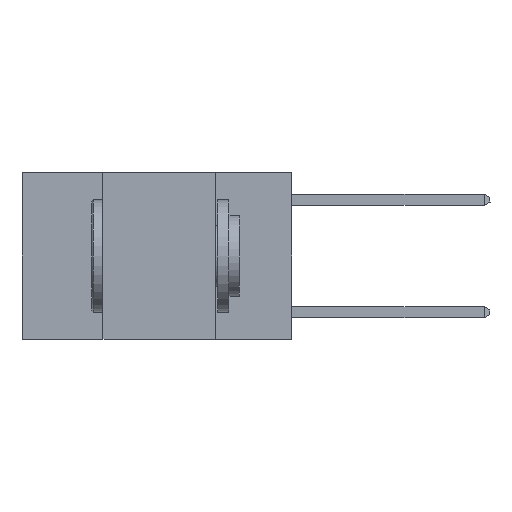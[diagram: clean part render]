
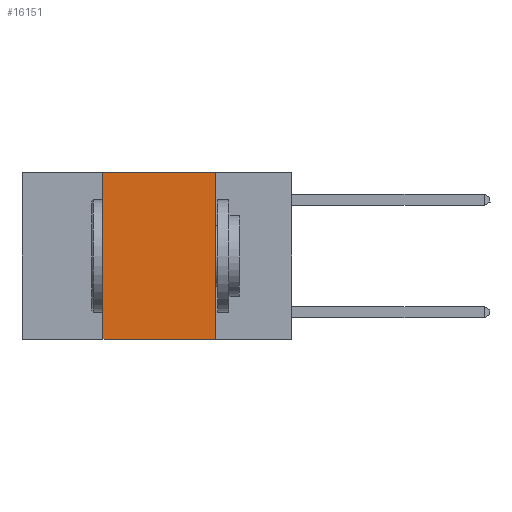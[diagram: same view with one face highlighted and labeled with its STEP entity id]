
A CAD part, left-side view. The second image highlights one B-rep face of the part: STEP entity #16151.
In plain terms, the highlighted planar face has unit normal (-1, 0, 0).
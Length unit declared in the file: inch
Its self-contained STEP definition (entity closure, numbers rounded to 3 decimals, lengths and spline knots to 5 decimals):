
#227 = ORIENTED_EDGE ( 'NONE', *, *, #9676, .F. ) ;
#1052 = VERTEX_POINT ( 'NONE', #8593 ) ;
#2266 = ORIENTED_EDGE ( 'NONE', *, *, #19657, .T. ) ;
#2409 = LINE ( 'NONE', #2533, #6175 ) ;
#2533 = CARTESIAN_POINT ( 'NONE',  ( 0., 0.6, -0.37 ) ) ;
#2713 = PLANE ( 'NONE',  #11467 ) ;
#2924 = CARTESIAN_POINT ( 'NONE',  ( 0., 0.42, 0. ) ) ;
#3151 = EDGE_CURVE ( 'NONE', #14523, #10203, #10865, .T. ) ;
#4199 = VECTOR ( 'NONE', #16200, 39.37008 ) ;
#5123 = CARTESIAN_POINT ( 'NONE',  ( 0., 0.42, 0. ) ) ;
#5180 = CARTESIAN_POINT ( 'NONE',  ( 0., 0.6, 0. ) ) ;
#5935 = DIRECTION ( 'NONE',  ( 1., 0., 0. ) ) ;
#6175 = VECTOR ( 'NONE', #15221, 39.37008 ) ;
#7619 = VERTEX_POINT ( 'NONE', #17030 ) ;
#7912 = LINE ( 'NONE', #5180, #4199 ) ;
#8593 = CARTESIAN_POINT ( 'NONE',  ( 0., 0.17, -0.37 ) ) ;
#9147 = VECTOR ( 'NONE', #14318, 39.37008 ) ;
#9570 = CARTESIAN_POINT ( 'NONE',  ( 0., 0.17, 0. ) ) ;
#9676 = EDGE_CURVE ( 'NONE', #7619, #1052, #13333, .T. ) ;
#10203 = VERTEX_POINT ( 'NONE', #2924 ) ;
#10865 = LINE ( 'NONE', #5123, #14537 ) ;
#11242 = EDGE_LOOP ( 'NONE', ( #227, #12951, #13444, #2266 ) ) ;
#11467 = AXIS2_PLACEMENT_3D ( 'NONE', #13826, #5935, #17010 ) ;
#12386 = CARTESIAN_POINT ( 'NONE',  ( 0., 0.42, -0.37 ) ) ;
#12951 = ORIENTED_EDGE ( 'NONE', *, *, #19443, .F. ) ;
#13333 = LINE ( 'NONE', #9570, #9147 ) ;
#13444 = ORIENTED_EDGE ( 'NONE', *, *, #3151, .F. ) ;
#13826 = CARTESIAN_POINT ( 'NONE',  ( 0., 0.6, 0. ) ) ;
#14318 = DIRECTION ( 'NONE',  ( 0., 0., -1. ) ) ;
#14523 = VERTEX_POINT ( 'NONE', #12386 ) ;
#14537 = VECTOR ( 'NONE', #16149, 39.37008 ) ;
#15221 = DIRECTION ( 'NONE',  ( 0., -1., 0. ) ) ;
#16149 = DIRECTION ( 'NONE',  ( 0., 0., 1. ) ) ;
#16151 = ADVANCED_FACE ( 'NONE', ( #16759 ), #2713, .F. ) ;
#16200 = DIRECTION ( 'NONE',  ( 0., -1., 0. ) ) ;
#16759 = FACE_OUTER_BOUND ( 'NONE', #11242, .T. ) ;
#17010 = DIRECTION ( 'NONE',  ( 0., 0., -1. ) ) ;
#17030 = CARTESIAN_POINT ( 'NONE',  ( 0., 0.17, 0. ) ) ;
#19443 = EDGE_CURVE ( 'NONE', #10203, #7619, #7912, .T. ) ;
#19657 = EDGE_CURVE ( 'NONE', #14523, #1052, #2409, .T. ) ;
